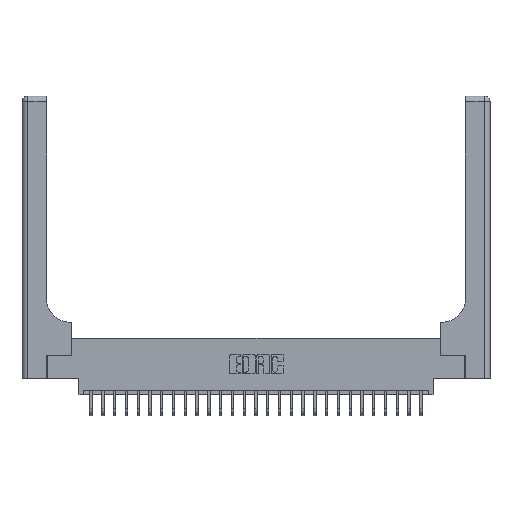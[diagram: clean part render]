
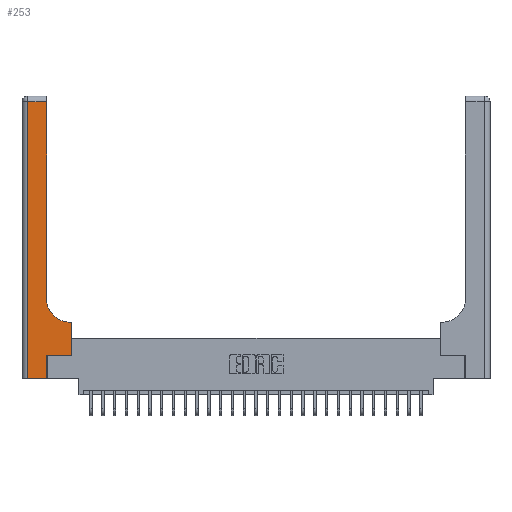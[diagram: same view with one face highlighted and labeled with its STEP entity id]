
A CAD part, top view. The second image highlights one B-rep face of the part: STEP entity #253.
In plain terms, the highlighted planar face has unit normal (0, 0, 1).
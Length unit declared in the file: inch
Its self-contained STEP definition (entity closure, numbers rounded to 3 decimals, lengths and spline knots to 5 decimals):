
#176 = DIRECTION ( 'NONE',  ( 0., 0., -1. ) ) ;
#253 = ADVANCED_FACE ( 'NONE', ( #17069 ), #10691, .F. ) ;
#405 = LINE ( 'NONE', #5376, #17596 ) ;
#655 = ORIENTED_EDGE ( 'NONE', *, *, #3356, .T. ) ;
#1580 = EDGE_CURVE ( 'NONE', #13793, #7147, #11384, .T. ) ;
#1929 = CARTESIAN_POINT ( 'NONE',  ( 0.528, 0.25, 0.37 ) ) ;
#2554 = LINE ( 'NONE', #26264, #12293 ) ;
#3297 = DIRECTION ( 'NONE',  ( -1., 0., 0. ) ) ;
#3356 = EDGE_CURVE ( 'NONE', #25276, #4573, #2554, .T. ) ;
#3739 = CARTESIAN_POINT ( 'NONE',  ( 0.265, 0.25, 0.37 ) ) ;
#4573 = VERTEX_POINT ( 'NONE', #24755 ) ;
#4983 = DIRECTION ( 'NONE',  ( 1., 0., 0. ) ) ;
#5376 = CARTESIAN_POINT ( 'NONE',  ( 0.26, 0.6, 0.37 ) ) ;
#6029 = VECTOR ( 'NONE', #11350, 39.37008 ) ;
#6826 = CARTESIAN_POINT ( 'NONE',  ( 0.528, 0.25, 0.37 ) ) ;
#7147 = VERTEX_POINT ( 'NONE', #3739 ) ;
#7480 = CARTESIAN_POINT ( 'NONE',  ( 0., 3., 0.37 ) ) ;
#8142 = EDGE_CURVE ( 'NONE', #22781, #25276, #24110, .T. ) ;
#8204 = CARTESIAN_POINT ( 'NONE',  ( 0.265, 0., 0.37 ) ) ;
#8372 = DIRECTION ( 'NONE',  ( 0., 1., 0. ) ) ;
#8867 = EDGE_CURVE ( 'NONE', #4573, #13793, #14650, .T. ) ;
#9101 = VERTEX_POINT ( 'NONE', #21210 ) ;
#9210 = ORIENTED_EDGE ( 'NONE', *, *, #21397, .T. ) ;
#9476 = LINE ( 'NONE', #24146, #15545 ) ;
#9888 = ORIENTED_EDGE ( 'NONE', *, *, #26849, .T. ) ;
#10691 = PLANE ( 'NONE',  #17260 ) ;
#10738 = EDGE_LOOP ( 'NONE', ( #23018, #25854, #655, #13624, #26184, #26311, #9210, #11991, #9888 ) ) ;
#11023 = EDGE_CURVE ( 'NONE', #7147, #21670, #9476, .T. ) ;
#11309 = DIRECTION ( 'NONE',  ( 1., 0., 0. ) ) ;
#11350 = DIRECTION ( 'NONE',  ( 0., 1., 0. ) ) ;
#11384 = LINE ( 'NONE', #8204, #23857 ) ;
#11819 = DIRECTION ( 'NONE',  ( 0., 0., -1. ) ) ;
#11841 = DIRECTION ( 'NONE',  ( -1., 0., 0. ) ) ;
#11991 = ORIENTED_EDGE ( 'NONE', *, *, #15892, .T. ) ;
#12293 = VECTOR ( 'NONE', #26095, 39.37008 ) ;
#13087 = CARTESIAN_POINT ( 'NONE',  ( 0.51, 0.85, 0.37 ) ) ;
#13386 = CARTESIAN_POINT ( 'NONE',  ( 0., 0., 0.37 ) ) ;
#13492 = CARTESIAN_POINT ( 'NONE',  ( 0.265, 0., 0.37 ) ) ;
#13624 = ORIENTED_EDGE ( 'NONE', *, *, #8867, .T. ) ;
#13793 = VERTEX_POINT ( 'NONE', #13492 ) ;
#13840 = CIRCLE ( 'NONE', #25038, 0.25 ) ;
#14006 = VERTEX_POINT ( 'NONE', #24553 ) ;
#14650 = LINE ( 'NONE', #13386, #17348 ) ;
#15371 = DIRECTION ( 'NONE',  ( 1., 0., 0. ) ) ;
#15545 = VECTOR ( 'NONE', #4983, 39.37008 ) ;
#15887 = CARTESIAN_POINT ( 'NONE',  ( 0., 2.94, 0.37 ) ) ;
#15892 = EDGE_CURVE ( 'NONE', #14006, #9101, #405, .T. ) ;
#16815 = CARTESIAN_POINT ( 'NONE',  ( 0.26, 2.94, 0.37 ) ) ;
#17069 = FACE_OUTER_BOUND ( 'NONE', #10738, .T. ) ;
#17260 = AXIS2_PLACEMENT_3D ( 'NONE', #7480, #11819, #3297 ) ;
#17264 = VERTEX_POINT ( 'NONE', #22732 ) ;
#17348 = VECTOR ( 'NONE', #11309, 39.37008 ) ;
#17596 = VECTOR ( 'NONE', #11841, 39.37008 ) ;
#18396 = VECTOR ( 'NONE', #22556, 39.37008 ) ;
#18937 = LINE ( 'NONE', #19392, #20283 ) ;
#19392 = CARTESIAN_POINT ( 'NONE',  ( 0.26, 3., 0.37 ) ) ;
#20283 = VECTOR ( 'NONE', #8372, 39.37008 ) ;
#21210 = CARTESIAN_POINT ( 'NONE',  ( 0.51, 0.6, 0.37 ) ) ;
#21397 = EDGE_CURVE ( 'NONE', #21670, #14006, #21867, .T. ) ;
#21670 = VERTEX_POINT ( 'NONE', #1929 ) ;
#21867 = LINE ( 'NONE', #6826, #6029 ) ;
#22363 = CARTESIAN_POINT ( 'NONE',  ( 0.06, 2.94, 0.37 ) ) ;
#22556 = DIRECTION ( 'NONE',  ( -1., 0., 0. ) ) ;
#22732 = CARTESIAN_POINT ( 'NONE',  ( 0.26, 0.85, 0.37 ) ) ;
#22781 = VERTEX_POINT ( 'NONE', #16815 ) ;
#23018 = ORIENTED_EDGE ( 'NONE', *, *, #26267, .T. ) ;
#23857 = VECTOR ( 'NONE', #25284, 39.37008 ) ;
#24110 = LINE ( 'NONE', #15887, #18396 ) ;
#24146 = CARTESIAN_POINT ( 'NONE',  ( 0.265, 0.25, 0.37 ) ) ;
#24553 = CARTESIAN_POINT ( 'NONE',  ( 0.528, 0.6, 0.37 ) ) ;
#24755 = CARTESIAN_POINT ( 'NONE',  ( 0.06, 0., 0.37 ) ) ;
#25038 = AXIS2_PLACEMENT_3D ( 'NONE', #13087, #176, #15371 ) ;
#25276 = VERTEX_POINT ( 'NONE', #22363 ) ;
#25284 = DIRECTION ( 'NONE',  ( 0., 1., 0. ) ) ;
#25854 = ORIENTED_EDGE ( 'NONE', *, *, #8142, .T. ) ;
#26095 = DIRECTION ( 'NONE',  ( 0., -1., 0. ) ) ;
#26184 = ORIENTED_EDGE ( 'NONE', *, *, #1580, .T. ) ;
#26264 = CARTESIAN_POINT ( 'NONE',  ( 0.06, 3., 0.37 ) ) ;
#26267 = EDGE_CURVE ( 'NONE', #17264, #22781, #18937, .T. ) ;
#26311 = ORIENTED_EDGE ( 'NONE', *, *, #11023, .T. ) ;
#26849 = EDGE_CURVE ( 'NONE', #9101, #17264, #13840, .T. ) ;
